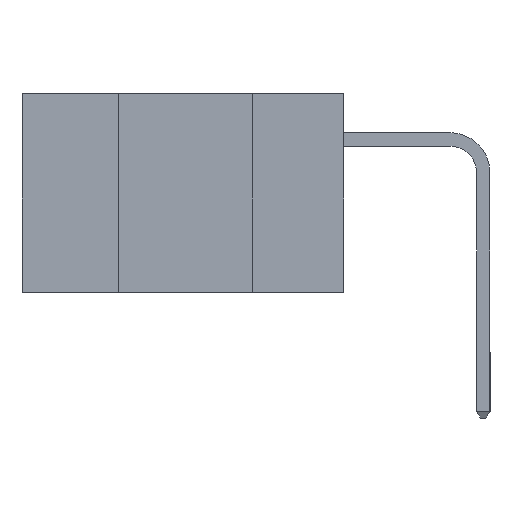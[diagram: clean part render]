
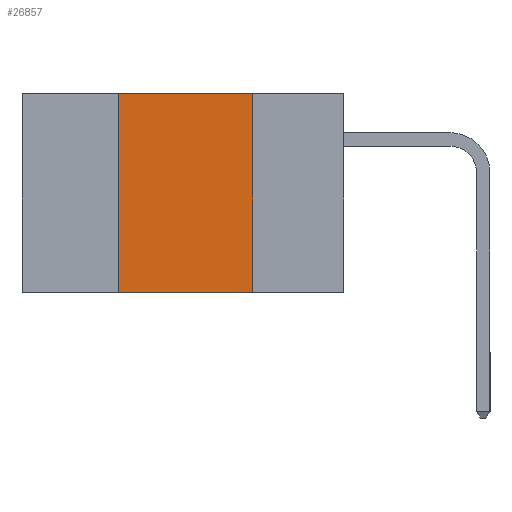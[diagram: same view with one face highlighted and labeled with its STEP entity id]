
A CAD part, left-side view. The second image highlights one B-rep face of the part: STEP entity #26857.
In plain terms, the highlighted planar face has unit normal (-1, 0, 0).
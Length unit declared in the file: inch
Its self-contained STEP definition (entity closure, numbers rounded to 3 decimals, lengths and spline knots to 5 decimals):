
#944 = PLANE ( 'NONE',  #7883 ) ;
#1005 = CARTESIAN_POINT ( 'NONE',  ( 0., 0.6, -0.37 ) ) ;
#1123 = DIRECTION ( 'NONE',  ( 0., 0., -1. ) ) ;
#2087 = EDGE_CURVE ( 'NONE', #19601, #11801, #7327, .T. ) ;
#3342 = VECTOR ( 'NONE', #27534, 39.37008 ) ;
#3399 = DIRECTION ( 'NONE',  ( 1., 0., 0. ) ) ;
#3837 = CARTESIAN_POINT ( 'NONE',  ( 0., 0.6, 0. ) ) ;
#4259 = CARTESIAN_POINT ( 'NONE',  ( 0., 0.17, 0. ) ) ;
#4303 = ORIENTED_EDGE ( 'NONE', *, *, #2087, .F. ) ;
#4386 = VERTEX_POINT ( 'NONE', #29878 ) ;
#5060 = VERTEX_POINT ( 'NONE', #4259 ) ;
#6062 = VECTOR ( 'NONE', #15268, 39.37008 ) ;
#7282 = EDGE_LOOP ( 'NONE', ( #17937, #24158, #4303, #10355 ) ) ;
#7327 = LINE ( 'NONE', #14592, #19176 ) ;
#7883 = AXIS2_PLACEMENT_3D ( 'NONE', #24746, #3399, #20047 ) ;
#10355 = ORIENTED_EDGE ( 'NONE', *, *, #18451, .T. ) ;
#11801 = VERTEX_POINT ( 'NONE', #27436 ) ;
#14592 = CARTESIAN_POINT ( 'NONE',  ( 0., 0.42, 0. ) ) ;
#15268 = DIRECTION ( 'NONE',  ( 0., -1., 0. ) ) ;
#15383 = CARTESIAN_POINT ( 'NONE',  ( 0., 0.17, 0. ) ) ;
#15832 = FACE_OUTER_BOUND ( 'NONE', #7282, .T. ) ;
#16464 = DIRECTION ( 'NONE',  ( 0., 0., 1. ) ) ;
#17100 = CARTESIAN_POINT ( 'NONE',  ( 0., 0.42, -0.37 ) ) ;
#17719 = LINE ( 'NONE', #15383, #18461 ) ;
#17937 = ORIENTED_EDGE ( 'NONE', *, *, #27625, .F. ) ;
#18451 = EDGE_CURVE ( 'NONE', #19601, #4386, #24288, .T. ) ;
#18461 = VECTOR ( 'NONE', #1123, 39.37008 ) ;
#19176 = VECTOR ( 'NONE', #16464, 39.37008 ) ;
#19601 = VERTEX_POINT ( 'NONE', #17100 ) ;
#20047 = DIRECTION ( 'NONE',  ( 0., 0., -1. ) ) ;
#22343 = LINE ( 'NONE', #3837, #3342 ) ;
#24158 = ORIENTED_EDGE ( 'NONE', *, *, #24477, .F. ) ;
#24288 = LINE ( 'NONE', #1005, #6062 ) ;
#24477 = EDGE_CURVE ( 'NONE', #11801, #5060, #22343, .T. ) ;
#24746 = CARTESIAN_POINT ( 'NONE',  ( 0., 0.6, 0. ) ) ;
#26857 = ADVANCED_FACE ( 'NONE', ( #15832 ), #944, .F. ) ;
#27436 = CARTESIAN_POINT ( 'NONE',  ( 0., 0.42, 0. ) ) ;
#27534 = DIRECTION ( 'NONE',  ( 0., -1., 0. ) ) ;
#27625 = EDGE_CURVE ( 'NONE', #5060, #4386, #17719, .T. ) ;
#29878 = CARTESIAN_POINT ( 'NONE',  ( 0., 0.17, -0.37 ) ) ;
